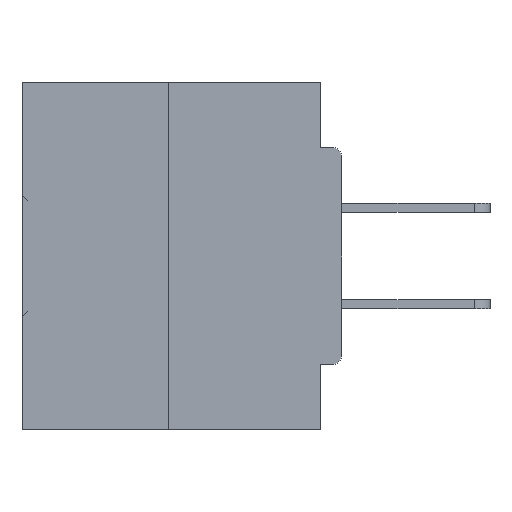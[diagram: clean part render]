
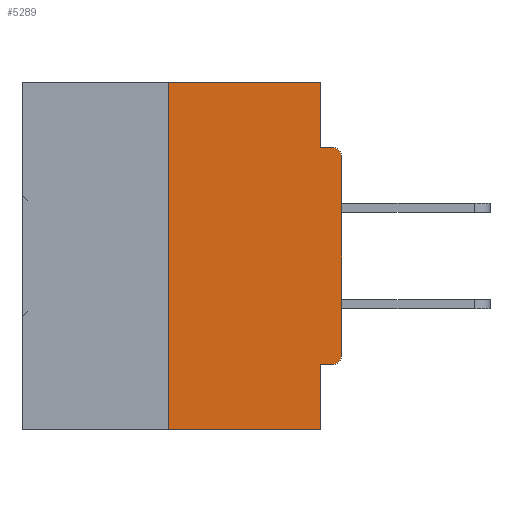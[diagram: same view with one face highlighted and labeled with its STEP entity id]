
A CAD part, left-side view. The second image highlights one B-rep face of the part: STEP entity #5289.
In plain terms, the highlighted planar face has unit normal (-1, 0, 0).
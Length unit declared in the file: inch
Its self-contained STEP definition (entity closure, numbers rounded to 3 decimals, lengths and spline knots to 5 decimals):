
#22 = ORIENTED_EDGE ( 'NONE', *, *, #41703, .T. ) ;
#266 = DIRECTION ( 'NONE',  ( 0., 0., -1. ) ) ;
#2318 = LINE ( 'NONE', #35901, #25183 ) ;
#3082 = CARTESIAN_POINT ( 'NONE',  ( 0., 0.46, 0. ) ) ;
#3950 = ORIENTED_EDGE ( 'NONE', *, *, #9220, .F. ) ;
#4115 = AXIS2_PLACEMENT_3D ( 'NONE', #31349, #27769, #6376 ) ;
#4964 = EDGE_CURVE ( 'NONE', #21995, #16660, #24755, .T. ) ;
#5205 = DIRECTION ( 'NONE',  ( 0., 0., -1. ) ) ;
#5289 = ADVANCED_FACE ( 'NONE', ( #20819 ), #9352, .F. ) ;
#5884 = ORIENTED_EDGE ( 'NONE', *, *, #7596, .F. ) ;
#6376 = DIRECTION ( 'NONE',  ( 0., 0., -1. ) ) ;
#6483 = CARTESIAN_POINT ( 'NONE',  ( 0., 0.031, -0.4065 ) ) ;
#7596 = EDGE_CURVE ( 'NONE', #35398, #11625, #36294, .T. ) ;
#8376 = VERTEX_POINT ( 'NONE', #37896 ) ;
#8737 = ORIENTED_EDGE ( 'NONE', *, *, #4964, .T. ) ;
#9046 = CARTESIAN_POINT ( 'NONE',  ( 0., 0.015, -0.4065 ) ) ;
#9220 = EDGE_CURVE ( 'NONE', #29953, #29804, #15429, .T. ) ;
#9352 = PLANE ( 'NONE',  #4115 ) ;
#10646 = EDGE_CURVE ( 'NONE', #33135, #21995, #15897, .T. ) ;
#10976 = VERTEX_POINT ( 'NONE', #33842 ) ;
#11625 = VERTEX_POINT ( 'NONE', #30618 ) ;
#15429 = LINE ( 'NONE', #21534, #29965 ) ;
#15873 = CIRCLE ( 'NONE', #46178, 0.015 ) ;
#15897 = CIRCLE ( 'NONE', #43222, 0.015 ) ;
#15952 = CARTESIAN_POINT ( 'NONE',  ( 0., 0.25, 0. ) ) ;
#15963 = CARTESIAN_POINT ( 'NONE',  ( 0., 0.031, 0. ) ) ;
#16043 = ORIENTED_EDGE ( 'NONE', *, *, #27364, .F. ) ;
#16660 = VERTEX_POINT ( 'NONE', #36059 ) ;
#17823 = ORIENTED_EDGE ( 'NONE', *, *, #10646, .T. ) ;
#18065 = DIRECTION ( 'NONE',  ( -1., 0., 0. ) ) ;
#19264 = CARTESIAN_POINT ( 'NONE',  ( 0., 0.031, -0.0935 ) ) ;
#19278 = CARTESIAN_POINT ( 'NONE',  ( 0., 0.015, -0.1085 ) ) ;
#19778 = CARTESIAN_POINT ( 'NONE',  ( 0., 0., -0.0935 ) ) ;
#19824 = EDGE_CURVE ( 'NONE', #34554, #10976, #39986, .T. ) ;
#20160 = LINE ( 'NONE', #19778, #25740 ) ;
#20819 = FACE_OUTER_BOUND ( 'NONE', #41349, .T. ) ;
#20926 = CARTESIAN_POINT ( 'NONE',  ( 0., 0., -0.3915 ) ) ;
#21534 = CARTESIAN_POINT ( 'NONE',  ( 0., 0.031, 0. ) ) ;
#21995 = VERTEX_POINT ( 'NONE', #20926 ) ;
#24330 = EDGE_CURVE ( 'NONE', #33135, #35398, #40358, .T. ) ;
#24755 = LINE ( 'NONE', #27776, #34822 ) ;
#25183 = VECTOR ( 'NONE', #25900, 39.37008 ) ;
#25740 = VECTOR ( 'NONE', #26950, 39.37008 ) ;
#25900 = DIRECTION ( 'NONE',  ( 0., -1., 0. ) ) ;
#26051 = LINE ( 'NONE', #3082, #37215 ) ;
#26784 = VECTOR ( 'NONE', #41058, 39.37008 ) ;
#26878 = CARTESIAN_POINT ( 'NONE',  ( 0., 0.031, -0.5 ) ) ;
#26950 = DIRECTION ( 'NONE',  ( 0., -1., 0. ) ) ;
#27364 = EDGE_CURVE ( 'NONE', #10976, #29953, #26051, .T. ) ;
#27769 = DIRECTION ( 'NONE',  ( 1., 0., 0. ) ) ;
#27776 = CARTESIAN_POINT ( 'NONE',  ( 0., 0., 0. ) ) ;
#29292 = VECTOR ( 'NONE', #33940, 39.37008 ) ;
#29804 = VERTEX_POINT ( 'NONE', #19264 ) ;
#29953 = VERTEX_POINT ( 'NONE', #15963 ) ;
#29965 = VECTOR ( 'NONE', #31841, 39.37008 ) ;
#30618 = CARTESIAN_POINT ( 'NONE',  ( 0., 0.031, -0.5 ) ) ;
#30852 = VECTOR ( 'NONE', #31219, 39.37008 ) ;
#31219 = DIRECTION ( 'NONE',  ( 0., 1., 0. ) ) ;
#31349 = CARTESIAN_POINT ( 'NONE',  ( 0., 0.46, 0. ) ) ;
#31454 = CARTESIAN_POINT ( 'NONE',  ( 0., 0.25, -0.5 ) ) ;
#31841 = DIRECTION ( 'NONE',  ( 0., 0., -1. ) ) ;
#33135 = VERTEX_POINT ( 'NONE', #9046 ) ;
#33354 = DIRECTION ( 'NONE',  ( 0., -1., 0. ) ) ;
#33842 = CARTESIAN_POINT ( 'NONE',  ( 0., 0.25, 0. ) ) ;
#33940 = DIRECTION ( 'NONE',  ( 0., 0., 1. ) ) ;
#33963 = DIRECTION ( 'NONE',  ( -1., 0., 0. ) ) ;
#34213 = CARTESIAN_POINT ( 'NONE',  ( 0., 0., -0.4065 ) ) ;
#34554 = VERTEX_POINT ( 'NONE', #31454 ) ;
#34822 = VECTOR ( 'NONE', #41714, 39.37008 ) ;
#35398 = VERTEX_POINT ( 'NONE', #6483 ) ;
#35901 = CARTESIAN_POINT ( 'NONE',  ( 0., 0.46, -0.5 ) ) ;
#36059 = CARTESIAN_POINT ( 'NONE',  ( 0., 0., -0.1085 ) ) ;
#36294 = LINE ( 'NONE', #26878, #26784 ) ;
#37149 = ORIENTED_EDGE ( 'NONE', *, *, #19824, .F. ) ;
#37215 = VECTOR ( 'NONE', #33354, 39.37008 ) ;
#37330 = EDGE_CURVE ( 'NONE', #34554, #11625, #2318, .T. ) ;
#37896 = CARTESIAN_POINT ( 'NONE',  ( 0., 0.015, -0.0935 ) ) ;
#39466 = CARTESIAN_POINT ( 'NONE',  ( 0., 0.015, -0.3915 ) ) ;
#39986 = LINE ( 'NONE', #15952, #29292 ) ;
#40189 = ORIENTED_EDGE ( 'NONE', *, *, #37330, .T. ) ;
#40358 = LINE ( 'NONE', #34213, #30852 ) ;
#41058 = DIRECTION ( 'NONE',  ( 0., 0., -1. ) ) ;
#41349 = EDGE_LOOP ( 'NONE', ( #16043, #37149, #40189, #5884, #41500, #17823, #8737, #22, #41935, #3950 ) ) ;
#41500 = ORIENTED_EDGE ( 'NONE', *, *, #24330, .F. ) ;
#41703 = EDGE_CURVE ( 'NONE', #16660, #8376, #15873, .T. ) ;
#41714 = DIRECTION ( 'NONE',  ( 0., 0., 1. ) ) ;
#41935 = ORIENTED_EDGE ( 'NONE', *, *, #44402, .F. ) ;
#43222 = AXIS2_PLACEMENT_3D ( 'NONE', #39466, #18065, #266 ) ;
#44402 = EDGE_CURVE ( 'NONE', #29804, #8376, #20160, .T. ) ;
#46178 = AXIS2_PLACEMENT_3D ( 'NONE', #19278, #33963, #5205 ) ;
